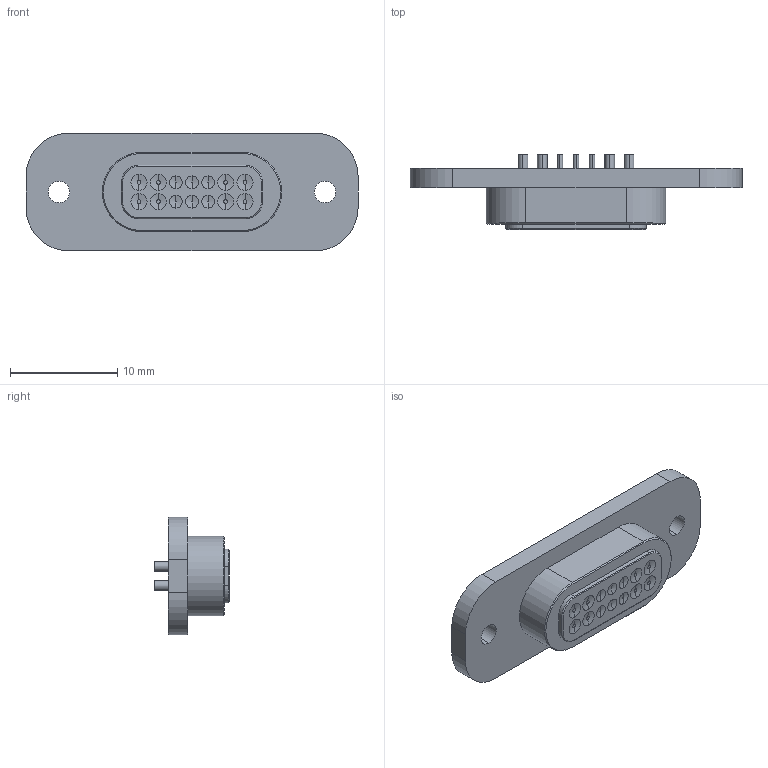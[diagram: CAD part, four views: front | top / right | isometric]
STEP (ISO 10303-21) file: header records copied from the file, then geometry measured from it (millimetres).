
FILE_DESCRIPTION (( 'STEP AP214' ), '1' );
FILE_NAME ('686A1451220113E.STEP', '2023-05-01T19:49:57', ( '' ), ( '' ), 'SwSTEP 2.0', 'SolidWorks 2020', '' );
FILE_SCHEMA (( 'AUTOMOTIVE_DESIGN' ));
Length unit declared in the file: millimetre
Products named in the file (1): 686A1451220113E
Bounding box: 31 x 7 x 11 mm (x, y, z)
Volume: 997.8 mm3; surface area: 1004.2 mm2
Topology: 1 solids, 1 shells, 166 faces, 348 edges, 228 vertices
Faces by surface type: cylinder 70, plane 62, cone 34
Entity records: 6386 total; most frequent: DIRECTION 884, CARTESIAN_POINT 743, ORIENTED_EDGE 696, AXIS2_PLACEMENT_3D 369, EDGE_CURVE 348, VERTEX_POINT 228, EDGE_LOOP 214, CIRCLE 202
